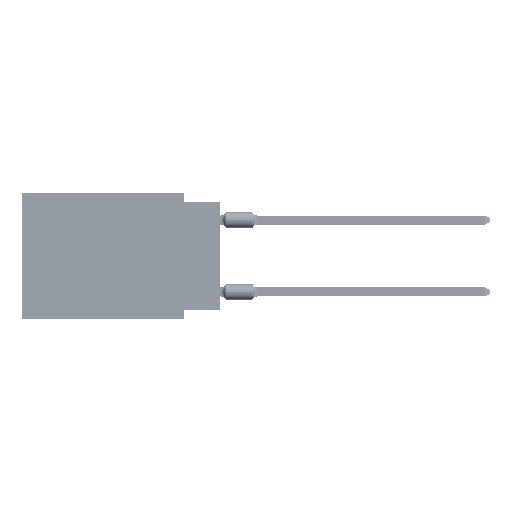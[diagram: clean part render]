
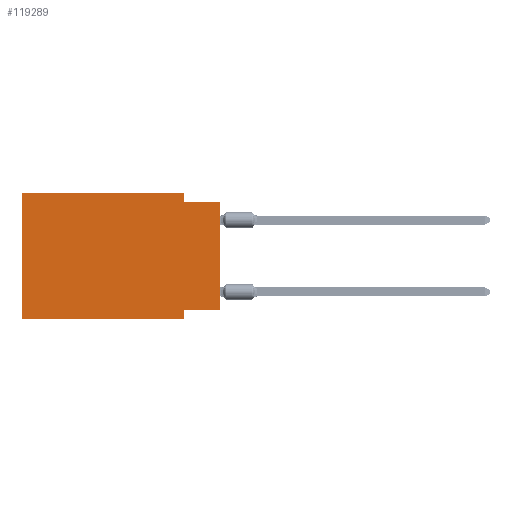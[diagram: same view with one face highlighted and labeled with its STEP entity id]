
A CAD part, left-side view. The second image highlights one B-rep face of the part: STEP entity #119289.
In plain terms, the highlighted planar face has unit normal (-1, 0, 0).
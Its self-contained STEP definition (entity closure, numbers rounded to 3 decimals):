
#3133 = DIRECTION ( 'NONE',  ( 0., -1., 0. ) ) ;
#4421 = EDGE_CURVE ( 'NONE', #12210, #91081, #79324, .T. ) ;
#11724 = DIRECTION ( 'NONE',  ( 0., 0., -1. ) ) ;
#12210 = VERTEX_POINT ( 'NONE', #55793 ) ;
#13340 = VERTEX_POINT ( 'NONE', #44427 ) ;
#13825 = ORIENTED_EDGE ( 'NONE', *, *, #39268, .F. ) ;
#16161 = DIRECTION ( 'NONE',  ( 0., 0., 1. ) ) ;
#16311 = EDGE_CURVE ( 'NONE', #115687, #12210, #91673, .T. ) ;
#17391 = CARTESIAN_POINT ( 'NONE',  ( 0., 13.97, 0. ) ) ;
#19856 = VECTOR ( 'NONE', #16161, 1000. ) ;
#23431 = ORIENTED_EDGE ( 'NONE', *, *, #110090, .T. ) ;
#25399 = ORIENTED_EDGE ( 'NONE', *, *, #74504, .F. ) ;
#26306 = EDGE_CURVE ( 'NONE', #13340, #110890, #117069, .T. ) ;
#26472 = CARTESIAN_POINT ( 'NONE',  ( 0., 2.54, -8.89 ) ) ;
#26510 = FACE_OUTER_BOUND ( 'NONE', #74668, .T. ) ;
#26561 = CARTESIAN_POINT ( 'NONE',  ( 0., 2.54, -8.255 ) ) ;
#28120 = CARTESIAN_POINT ( 'NONE',  ( 0., 0., -0.635 ) ) ;
#28441 = CARTESIAN_POINT ( 'NONE',  ( 0., 13.97, 0. ) ) ;
#28451 = CARTESIAN_POINT ( 'NONE',  ( 0., 2.54, 0. ) ) ;
#30838 = VECTOR ( 'NONE', #33157, 1000. ) ;
#31332 = CARTESIAN_POINT ( 'NONE',  ( 0., 2.54, 0. ) ) ;
#33157 = DIRECTION ( 'NONE',  ( 0., -1., 0. ) ) ;
#33444 = VERTEX_POINT ( 'NONE', #26561 ) ;
#35769 = CARTESIAN_POINT ( 'NONE',  ( 0., 0., -8.255 ) ) ;
#36943 = EDGE_CURVE ( 'NONE', #33444, #49606, #115014, .T. ) ;
#39268 = EDGE_CURVE ( 'NONE', #67066, #33444, #50844, .T. ) ;
#42340 = DIRECTION ( 'NONE',  ( 0., 1., 0. ) ) ;
#44427 = CARTESIAN_POINT ( 'NONE',  ( 0., 13.97, -8.89 ) ) ;
#44923 = LINE ( 'NONE', #28441, #94257 ) ;
#48759 = LINE ( 'NONE', #57250, #114189 ) ;
#49606 = VERTEX_POINT ( 'NONE', #26472 ) ;
#50844 = LINE ( 'NONE', #88502, #58967 ) ;
#54451 = DIRECTION ( 'NONE',  ( 1., 0., 0. ) ) ;
#55793 = CARTESIAN_POINT ( 'NONE',  ( 0., 2.54, -0.635 ) ) ;
#56440 = LINE ( 'NONE', #94085, #65097 ) ;
#57250 = CARTESIAN_POINT ( 'NONE',  ( 0., 13.97, -8.89 ) ) ;
#58967 = VECTOR ( 'NONE', #42340, 1000. ) ;
#59530 = EDGE_CURVE ( 'NONE', #67066, #91081, #56440, .T. ) ;
#59687 = ORIENTED_EDGE ( 'NONE', *, *, #16311, .F. ) ;
#63553 = PLANE ( 'NONE',  #110438 ) ;
#65097 = VECTOR ( 'NONE', #84970, 1000. ) ;
#66096 = ORIENTED_EDGE ( 'NONE', *, *, #36943, .F. ) ;
#67066 = VERTEX_POINT ( 'NONE', #35769 ) ;
#74504 = EDGE_CURVE ( 'NONE', #110890, #115687, #44923, .T. ) ;
#74668 = EDGE_LOOP ( 'NONE', ( #96793, #100049, #59687, #25399, #85315, #23431, #66096, #13825 ) ) ;
#76739 = CARTESIAN_POINT ( 'NONE',  ( 0., 2.54, -8.89 ) ) ;
#79324 = LINE ( 'NONE', #116419, #30838 ) ;
#81058 = VECTOR ( 'NONE', #102570, 1000. ) ;
#81978 = DIRECTION ( 'NONE',  ( 0., -1., 0. ) ) ;
#84970 = DIRECTION ( 'NONE',  ( 0., 0., 1. ) ) ;
#85315 = ORIENTED_EDGE ( 'NONE', *, *, #26306, .F. ) ;
#88502 = CARTESIAN_POINT ( 'NONE',  ( 0., 0., -8.255 ) ) ;
#91081 = VERTEX_POINT ( 'NONE', #28120 ) ;
#91512 = DIRECTION ( 'NONE',  ( 0., 0., -1. ) ) ;
#91673 = LINE ( 'NONE', #28451, #81058 ) ;
#94011 = CARTESIAN_POINT ( 'NONE',  ( 0., 13.97, 0. ) ) ;
#94085 = CARTESIAN_POINT ( 'NONE',  ( 0., 0., 0. ) ) ;
#94257 = VECTOR ( 'NONE', #81978, 1000. ) ;
#95657 = VECTOR ( 'NONE', #11724, 1000. ) ;
#96793 = ORIENTED_EDGE ( 'NONE', *, *, #59530, .T. ) ;
#100049 = ORIENTED_EDGE ( 'NONE', *, *, #4421, .F. ) ;
#102570 = DIRECTION ( 'NONE',  ( 0., 0., -1. ) ) ;
#110090 = EDGE_CURVE ( 'NONE', #13340, #49606, #48759, .T. ) ;
#110438 = AXIS2_PLACEMENT_3D ( 'NONE', #17391, #54451, #91512 ) ;
#110890 = VERTEX_POINT ( 'NONE', #94011 ) ;
#114189 = VECTOR ( 'NONE', #3133, 1000. ) ;
#115014 = LINE ( 'NONE', #76739, #95657 ) ;
#115273 = CARTESIAN_POINT ( 'NONE',  ( 0., 13.97, 0. ) ) ;
#115687 = VERTEX_POINT ( 'NONE', #31332 ) ;
#116419 = CARTESIAN_POINT ( 'NONE',  ( 0., 0., -0.635 ) ) ;
#117069 = LINE ( 'NONE', #115273, #19856 ) ;
#119289 = ADVANCED_FACE ( 'NONE', ( #26510 ), #63553, .F. ) ;
